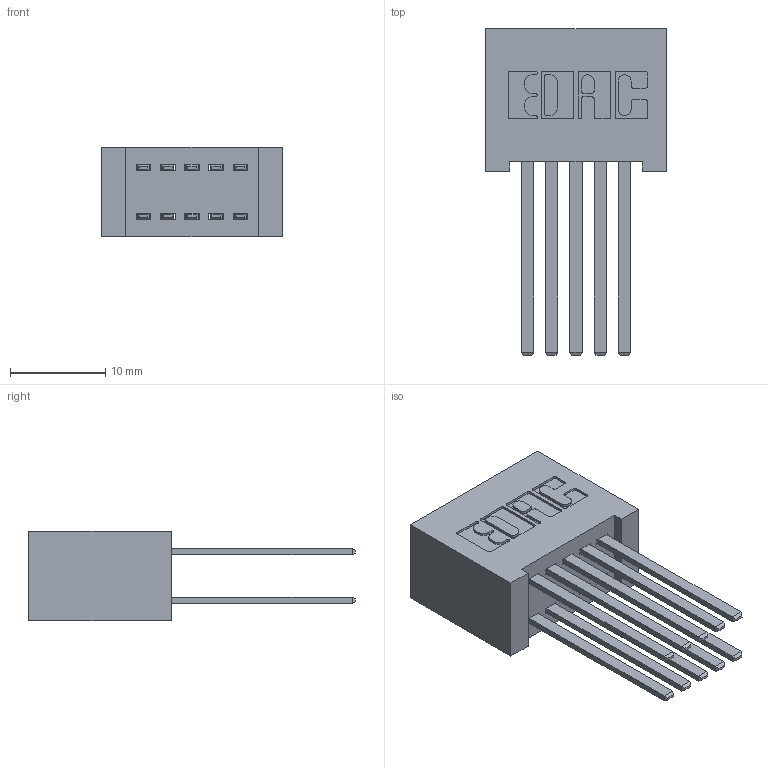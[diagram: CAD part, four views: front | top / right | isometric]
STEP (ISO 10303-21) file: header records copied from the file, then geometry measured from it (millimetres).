
FILE_DESCRIPTION (( 'STEP AP203' ), '1' );
FILE_NAME ('392-010-544-201.STEP', '2019-10-05T01:04:55', ( '' ), ( '' ), 'SwSTEP 2.0', 'SolidWorks 2016', '' );
FILE_SCHEMA (( 'CONFIG_CONTROL_DESIGN' ));
Length unit declared in the file: inch
Products named in the file (3): 342 Part_Lugless; 345-292-001_345-293-144; 392-010-544-201
Assembly tree (11 placements, depth 2):
  392-010-544-201
    342 Part_Lugless
    345-292-001_345-293-144  x10
Bounding box: 18.95 x 34.3 x 9.4 mm (x, y, z)
Volume: 2107.1 mm3; surface area: 3352.5 mm2
Topology: 11 solids, 11 shells, 562 faces, 1645 edges, 1082 vertices
Faces by surface type: plane 382, cylinder 180
Entity records: 7409 total; most frequent: CARTESIAN_POINT 1266, ORIENTED_EDGE 1202, DIRECTION 1137, EDGE_CURVE 601, VECTOR 485, LINE 485, VERTEX_POINT 398, AXIS2_PLACEMENT_3D 326
